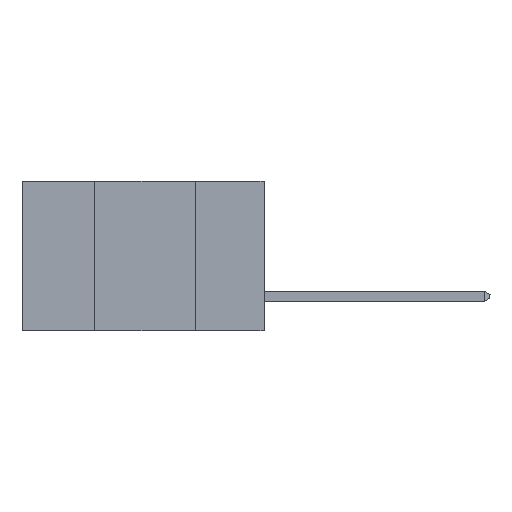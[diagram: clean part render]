
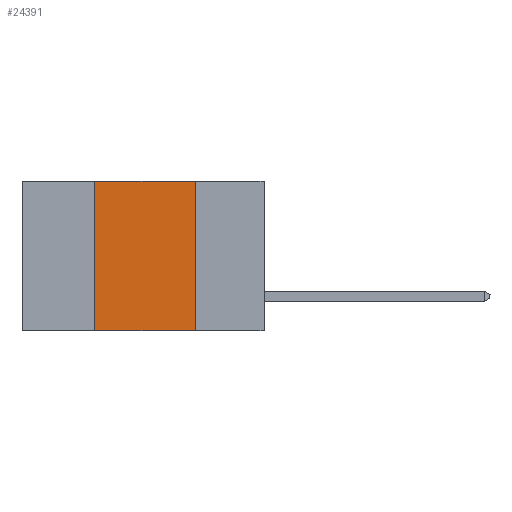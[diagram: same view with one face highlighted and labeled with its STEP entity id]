
A CAD part, left-side view. The second image highlights one B-rep face of the part: STEP entity #24391.
In plain terms, the highlighted planar face has unit normal (-1, 0, 0).
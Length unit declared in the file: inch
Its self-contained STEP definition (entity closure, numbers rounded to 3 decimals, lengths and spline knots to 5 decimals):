
#608 = ORIENTED_EDGE ( 'NONE', *, *, #6952, .F. ) ;
#973 = LINE ( 'NONE', #4214, #5849 ) ;
#1672 = PLANE ( 'NONE',  #6409 ) ;
#2048 = LINE ( 'NONE', #7810, #28843 ) ;
#2412 = EDGE_CURVE ( 'NONE', #25344, #3925, #973, .T. ) ;
#2928 = CARTESIAN_POINT ( 'NONE',  ( 0., 0.17, 0. ) ) ;
#3925 = VERTEX_POINT ( 'NONE', #5808 ) ;
#4214 = CARTESIAN_POINT ( 'NONE',  ( 0., 0.42, 0. ) ) ;
#5808 = CARTESIAN_POINT ( 'NONE',  ( 0., 0.42, 0. ) ) ;
#5849 = VECTOR ( 'NONE', #6634, 39.37008 ) ;
#6005 = CARTESIAN_POINT ( 'NONE',  ( 0., 0.6, 0. ) ) ;
#6295 = LINE ( 'NONE', #6005, #24495 ) ;
#6409 = AXIS2_PLACEMENT_3D ( 'NONE', #13496, #15866, #18433 ) ;
#6634 = DIRECTION ( 'NONE',  ( 0., 0., 1. ) ) ;
#6952 = EDGE_CURVE ( 'NONE', #3925, #22575, #6295, .T. ) ;
#7810 = CARTESIAN_POINT ( 'NONE',  ( 0., 0.17, 0. ) ) ;
#10783 = CARTESIAN_POINT ( 'NONE',  ( 0., 0.6, -0.37 ) ) ;
#12439 = EDGE_CURVE ( 'NONE', #25344, #24071, #15777, .T. ) ;
#13496 = CARTESIAN_POINT ( 'NONE',  ( 0., 0.6, 0. ) ) ;
#13853 = ORIENTED_EDGE ( 'NONE', *, *, #2412, .F. ) ;
#15777 = LINE ( 'NONE', #10783, #17996 ) ;
#15866 = DIRECTION ( 'NONE',  ( 1., 0., 0. ) ) ;
#16679 = FACE_OUTER_BOUND ( 'NONE', #18572, .T. ) ;
#17996 = VECTOR ( 'NONE', #20110, 39.37008 ) ;
#18425 = CARTESIAN_POINT ( 'NONE',  ( 0., 0.42, -0.37 ) ) ;
#18433 = DIRECTION ( 'NONE',  ( 0., 0., -1. ) ) ;
#18572 = EDGE_LOOP ( 'NONE', ( #25989, #608, #13853, #22089 ) ) ;
#20110 = DIRECTION ( 'NONE',  ( 0., -1., 0. ) ) ;
#22089 = ORIENTED_EDGE ( 'NONE', *, *, #12439, .T. ) ;
#22575 = VERTEX_POINT ( 'NONE', #2928 ) ;
#24071 = VERTEX_POINT ( 'NONE', #24099 ) ;
#24099 = CARTESIAN_POINT ( 'NONE',  ( 0., 0.17, -0.37 ) ) ;
#24391 = ADVANCED_FACE ( 'NONE', ( #16679 ), #1672, .F. ) ;
#24495 = VECTOR ( 'NONE', #29533, 39.37008 ) ;
#25344 = VERTEX_POINT ( 'NONE', #18425 ) ;
#25989 = ORIENTED_EDGE ( 'NONE', *, *, #26517, .F. ) ;
#26517 = EDGE_CURVE ( 'NONE', #22575, #24071, #2048, .T. ) ;
#26785 = DIRECTION ( 'NONE',  ( 0., 0., -1. ) ) ;
#28843 = VECTOR ( 'NONE', #26785, 39.37008 ) ;
#29533 = DIRECTION ( 'NONE',  ( 0., -1., 0. ) ) ;
